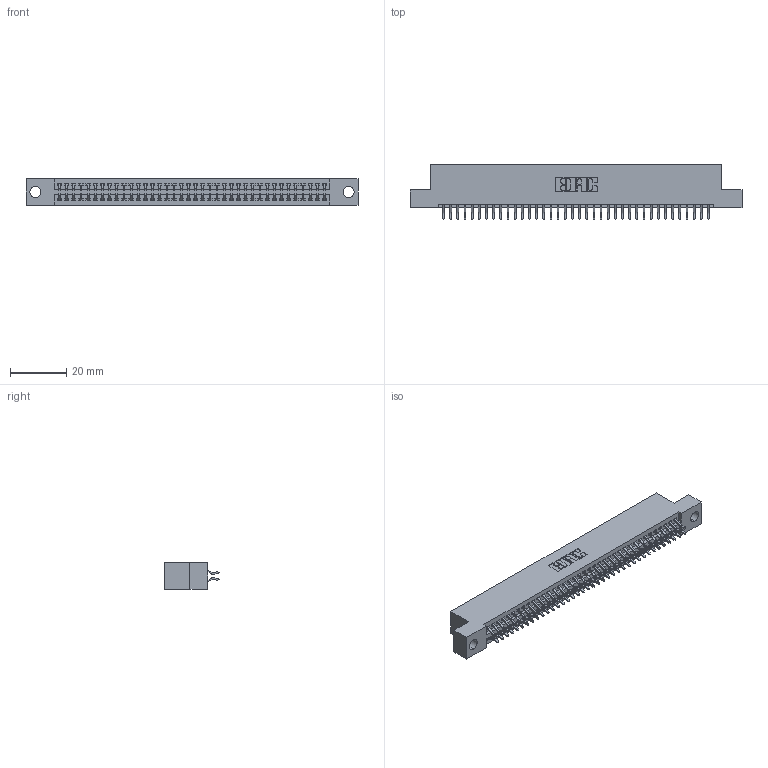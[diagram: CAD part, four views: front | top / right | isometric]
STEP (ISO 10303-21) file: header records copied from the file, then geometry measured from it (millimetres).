
FILE_DESCRIPTION (( 'STEP AP203' ), '1' );
FILE_NAME ('395-076-556-204.STEP', '2021-06-17T06:12:26', ( '' ), ( '' ), 'SwSTEP 2.0', 'SolidWorks 2020', '' );
FILE_SCHEMA (( 'CONFIG_CONTROL_DESIGN' ));
Length unit declared in the file: inch
Products named in the file (3): 395-076-556-204; 345-292-001_556 Tail; 345 Part_Flush Mounting Lugs - 0.156 Dia-TI
Assembly tree (77 placements, depth 2):
  395-076-556-204
    345 Part_Flush Mounting Lugs - 0.156 Dia-TI
    345-292-001_556 Tail  x76
Bounding box: 117.73 x 19.24 x 9.4 mm (x, y, z)
Volume: 11290.2 mm3; surface area: 16396.4 mm2
Topology: 77 solids, 77 shells, 4396 faces, 13069 edges, 8610 vertices
Faces by surface type: plane 2906, cylinder 1490
Entity records: 30993 total; most frequent: CARTESIAN_POINT 5218, ORIENTED_EDGE 5138, DIRECTION 4593, EDGE_CURVE 2569, VECTOR 2277, LINE 2277, VERTEX_POINT 1710, AXIS2_PLACEMENT_3D 1158
